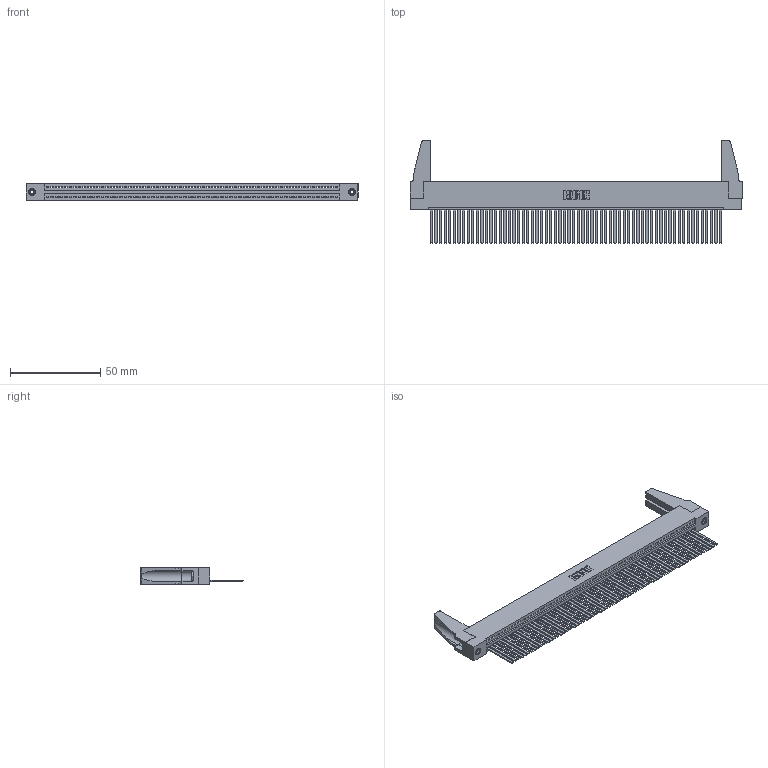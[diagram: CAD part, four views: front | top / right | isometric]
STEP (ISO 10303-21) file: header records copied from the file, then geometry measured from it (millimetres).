
FILE_DESCRIPTION (( 'STEP AP203' ), '1' );
FILE_NAME ('395-064-544-188.STEP', '2019-10-25T03:18:10', ( '' ), ( '' ), 'SwSTEP 2.0', 'SolidWorks 2016', '' );
FILE_SCHEMA (( 'CONFIG_CONTROL_DESIGN' ));
Length unit declared in the file: inch
Products named in the file (5): 345-220-078_345-220-088; 395-064-544-188; 345-292-001_345-293-144; 345 Part_Flush Mounting Lugs - 0.156 Dia-TH; 345-250-001_345-250-001-102
Assembly tree (69 placements, depth 2):
  395-064-544-188
    345 Part_Flush Mounting Lugs - 0.156 Dia-TH
    345-292-001_345-293-144  x64
    345-250-001_345-250-001-102  x2
    345-220-078_345-220-088  x2
Bounding box: 183.79 x 56.82 x 9.4 mm (x, y, z)
Volume: 21630.9 mm3; surface area: 30076.7 mm2
Topology: 69 solids, 69 shells, 3578 faces, 10767 edges, 7082 vertices
Faces by surface type: plane 2456, cylinder 1106, cone 12, torus 4
Entity records: 47170 total; most frequent: CARTESIAN_POINT 8158, ORIENTED_EDGE 8116, DIRECTION 7098, EDGE_CURVE 4058, VECTOR 3632, LINE 3632, VERTEX_POINT 2698, AXIS2_PLACEMENT_3D 1733
